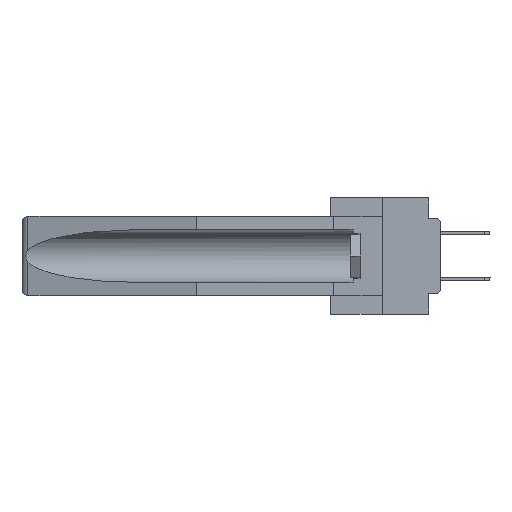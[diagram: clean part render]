
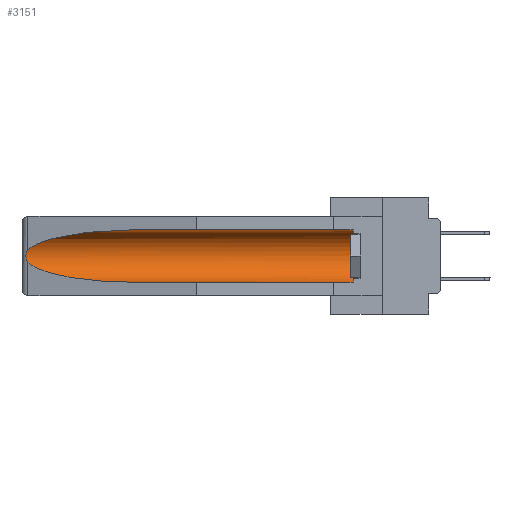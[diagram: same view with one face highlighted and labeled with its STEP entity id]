
A CAD part, left-side view. The second image highlights one B-rep face of the part: STEP entity #3151.
In plain terms, the highlighted cylindrical face has radius 2.857 mm (diameter 5.715 mm), a partial arc.
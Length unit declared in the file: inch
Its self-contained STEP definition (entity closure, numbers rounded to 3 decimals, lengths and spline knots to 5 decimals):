
#174 = FACE_OUTER_BOUND ( 'NONE', #4707, .T. ) ;
#1026 = CARTESIAN_POINT ( 'NONE',  ( 0.155, 1.07973, -0.284 ) ) ;
#1470 = CARTESIAN_POINT ( 'NONE',  ( 0.25451, 1.48313, -0.09465 ) ) ;
#1615 = CARTESIAN_POINT ( 'NONE',  ( 0.26537, 1.52718, -0.14972 ) ) ;
#1683 = CARTESIAN_POINT ( 'NONE',  ( 0.26537, 1.52718, -0.14972 ) ) ;
#1770 = ORIENTED_EDGE ( 'NONE', *, *, #12489, .F. ) ;
#2632 = CARTESIAN_POINT ( 'NONE',  ( 0.21114, 1.30732, -0.284 ) ) ;
#3151 = ADVANCED_FACE ( 'NONE', ( #174 ), #18383, .F. ) ;
#3643 = CARTESIAN_POINT ( 'NONE',  ( 0.26597, 1.5296, -0.19026 ) ) ;
#4301 = CARTESIAN_POINT ( 'NONE',  ( 0.155, -0.30754, -0.284 ) ) ;
#4475 = VECTOR ( 'NONE', #21361, 39.37008 ) ;
#4707 = EDGE_LOOP ( 'NONE', ( #30182, #17533, #20687, #1770, #25853, #11506 ) ) ;
#4872 = CARTESIAN_POINT ( 'NONE',  ( 0.26537, 1.52718, -0.19328 ) ) ;
#6323 = VECTOR ( 'NONE', #23231, 39.37008 ) ;
#10487 = VERTEX_POINT ( 'NONE', #1026 ) ;
#10905 = CARTESIAN_POINT ( 'NONE',  ( 0.155, 0.126, -0.059 ) ) ;
#11136 = EDGE_CURVE ( 'NONE', #16675, #23542, #28253, .T. ) ;
#11335 = CARTESIAN_POINT ( 'NONE',  ( 0.21114, 1.30732, -0.059 ) ) ;
#11506 = ORIENTED_EDGE ( 'NONE', *, *, #11136, .T. ) ;
#12073 = EDGE_CURVE ( 'NONE', #26150, #10487, #19718, .T. ) ;
#12279 = CIRCLE ( 'NONE', #21468, 0.1125 ) ;
#12286 = CARTESIAN_POINT ( 'NONE',  ( 0.25451, 1.48313, -0.24835 ) ) ;
#12489 = EDGE_CURVE ( 'NONE', #14839, #10487, #22676, .T. ) ;
#13303 = CARTESIAN_POINT ( 'NONE',  ( 0.2675, 1.53308, -0.16763 ) ) ;
#14839 = VERTEX_POINT ( 'NONE', #15547 ) ;
#15547 = CARTESIAN_POINT ( 'NONE',  ( 0.155, 0.126, -0.284 ) ) ;
#15621 = CARTESIAN_POINT ( 'NONE',  ( 0.155, -0.30754, -0.1715 ) ) ;
#15874 = DIRECTION ( 'NONE',  ( 0., 0., 1. ) ) ;
#15967 = AXIS2_PLACEMENT_3D ( 'NONE', #15621, #30422, #30532 ) ;
#16141 = CARTESIAN_POINT ( 'NONE',  ( 0.2675, 1.53308, -0.17534 ) ) ;
#16675 = VERTEX_POINT ( 'NONE', #10905 ) ;
#17533 = ORIENTED_EDGE ( 'NONE', *, *, #23207, .T. ) ;
#17585 = DIRECTION ( 'NONE',  ( 0., -1., 0. ) ) ;
#18383 = CYLINDRICAL_SURFACE ( 'NONE', #15967, 0.1125 ) ;
#18497 = CARTESIAN_POINT ( 'NONE',  ( 0.26654, 1.53092, -0.15636 ) ) ;
#18605 = CARTESIAN_POINT ( 'NONE',  ( 0.26655, 1.53094, -0.18657 ) ) ;
#19718 =( BOUNDED_CURVE ( )  B_SPLINE_CURVE ( 3, ( #4872, #12286, #2632, #21825 ),
 .UNSPECIFIED., .F., .F. ) 
 B_SPLINE_CURVE_WITH_KNOTS ( ( 4, 4 ),
 ( 0.1948, 1.5708 ),
 .UNSPECIFIED. ) 
 CURVE ( )  GEOMETRIC_REPRESENTATION_ITEM ( )  RATIONAL_B_SPLINE_CURVE ( ( 1., 0.848, 0.848, 1. ) ) 
 REPRESENTATION_ITEM ( '' )  );
#20687 = ORIENTED_EDGE ( 'NONE', *, *, #12073, .T. ) ;
#20994 = CARTESIAN_POINT ( 'NONE',  ( 0.26537, 1.52718, -0.19328 ) ) ;
#21063 = B_SPLINE_CURVE_WITH_KNOTS ( 'NONE', 3,
 ( #27770, #30530, #18497, #23340, #13303, #16141, #30218, #18605, #3643, #21123 ),
 .UNSPECIFIED., .F., .F.,
 ( 4, 2, 2, 2, 4 ),
 ( 0., 0.00029, 0.00058, 0.00087, 0.00117 ),
 .UNSPECIFIED. ) ;
#21116 = CARTESIAN_POINT ( 'NONE',  ( 0.155, -0.30754, -0.059 ) ) ;
#21123 = CARTESIAN_POINT ( 'NONE',  ( 0.26537, 1.52718, -0.19328 ) ) ;
#21361 = DIRECTION ( 'NONE',  ( 0., 1., 0. ) ) ;
#21468 = AXIS2_PLACEMENT_3D ( 'NONE', #30367, #17585, #15874 ) ;
#21825 = CARTESIAN_POINT ( 'NONE',  ( 0.155, 1.07973, -0.284 ) ) ;
#22070 = CARTESIAN_POINT ( 'NONE',  ( 0.155, 1.07973, -0.059 ) ) ;
#22676 = LINE ( 'NONE', #4301, #4475 ) ;
#23207 = EDGE_CURVE ( 'NONE', #30836, #26150, #21063, .T. ) ;
#23231 = DIRECTION ( 'NONE',  ( 0., 1., 0. ) ) ;
#23340 = CARTESIAN_POINT ( 'NONE',  ( 0.2673, 1.5327, -0.16383 ) ) ;
#23383 = CARTESIAN_POINT ( 'NONE',  ( 0.155, 1.07973, -0.059 ) ) ;
#23542 = VERTEX_POINT ( 'NONE', #22070 ) ;
#25853 = ORIENTED_EDGE ( 'NONE', *, *, #26503, .T. ) ;
#26150 = VERTEX_POINT ( 'NONE', #20994 ) ;
#26503 = EDGE_CURVE ( 'NONE', #14839, #16675, #12279, .T. ) ;
#27770 = CARTESIAN_POINT ( 'NONE',  ( 0.26537, 1.52718, -0.14972 ) ) ;
#28253 = LINE ( 'NONE', #21116, #6323 ) ;
#28598 =( BOUNDED_CURVE ( )  B_SPLINE_CURVE ( 3, ( #23383, #11335, #1470, #1683 ),
 .UNSPECIFIED., .F., .F. ) 
 B_SPLINE_CURVE_WITH_KNOTS ( ( 4, 4 ),
 ( 4.71239, 6.08839 ),
 .UNSPECIFIED. ) 
 CURVE ( )  GEOMETRIC_REPRESENTATION_ITEM ( )  RATIONAL_B_SPLINE_CURVE ( ( 1., 0.848, 0.848, 1. ) ) 
 REPRESENTATION_ITEM ( '' )  );
#28705 = EDGE_CURVE ( 'NONE', #23542, #30836, #28598, .T. ) ;
#30182 = ORIENTED_EDGE ( 'NONE', *, *, #28705, .T. ) ;
#30218 = CARTESIAN_POINT ( 'NONE',  ( 0.2673, 1.53269, -0.17917 ) ) ;
#30367 = CARTESIAN_POINT ( 'NONE',  ( 0.155, 0.126, -0.1715 ) ) ;
#30422 = DIRECTION ( 'NONE',  ( 0., 1., 0. ) ) ;
#30530 = CARTESIAN_POINT ( 'NONE',  ( 0.26597, 1.52961, -0.15275 ) ) ;
#30532 = DIRECTION ( 'NONE',  ( 0., 0., 1. ) ) ;
#30836 = VERTEX_POINT ( 'NONE', #1615 ) ;
